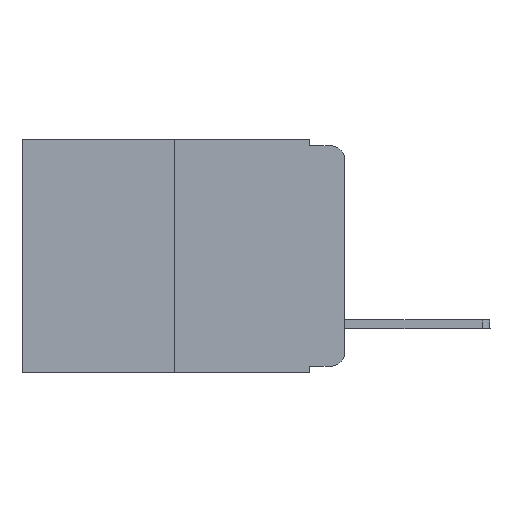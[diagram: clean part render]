
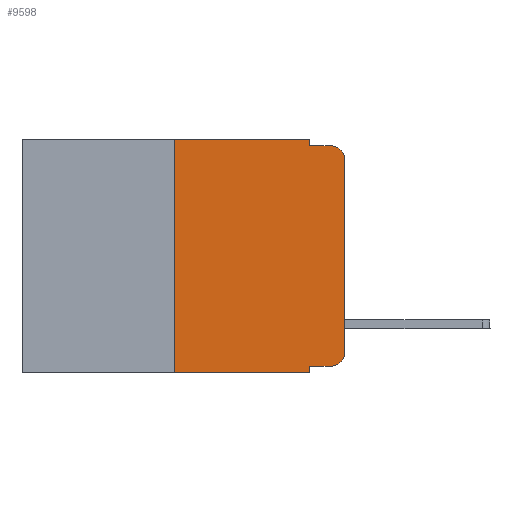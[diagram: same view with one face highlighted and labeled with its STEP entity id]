
A CAD part, left-side view. The second image highlights one B-rep face of the part: STEP entity #9598.
In plain terms, the highlighted planar face has unit normal (-1, 0, 0).
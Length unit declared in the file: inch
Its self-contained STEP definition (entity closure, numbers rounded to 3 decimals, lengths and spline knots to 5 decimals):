
#320 = CARTESIAN_POINT ( 'NONE',  ( 0., 0.02, -0.333 ) ) ;
#509 = ORIENTED_EDGE ( 'NONE', *, *, #8006, .T. ) ;
#600 = DIRECTION ( 'NONE',  ( 0., -1., 0. ) ) ;
#733 = DIRECTION ( 'NONE',  ( 0., 0., 1. ) ) ;
#1272 = AXIS2_PLACEMENT_3D ( 'NONE', #6115, #7047, #1819 ) ;
#1307 = CARTESIAN_POINT ( 'NONE',  ( 0., 0.051, 0. ) ) ;
#1331 = EDGE_CURVE ( 'NONE', #5371, #3654, #4336, .T. ) ;
#1522 = DIRECTION ( 'NONE',  ( 0., -1., 0. ) ) ;
#1611 = EDGE_CURVE ( 'NONE', #2599, #4344, #7031, .T. ) ;
#1660 = CARTESIAN_POINT ( 'NONE',  ( 0., 0.051, -0.01 ) ) ;
#1819 = DIRECTION ( 'NONE',  ( 0., 0., -1. ) ) ;
#1866 = LINE ( 'NONE', #10562, #9379 ) ;
#2234 = DIRECTION ( 'NONE',  ( 1., 0., 0. ) ) ;
#2406 = DIRECTION ( 'NONE',  ( 0., 0., -1. ) ) ;
#2551 = CARTESIAN_POINT ( 'NONE',  ( 0., 0., 0. ) ) ;
#2599 = VERTEX_POINT ( 'NONE', #320 ) ;
#3126 = CARTESIAN_POINT ( 'NONE',  ( 0., 0.473, 0. ) ) ;
#3312 = VECTOR ( 'NONE', #733, 39.37008 ) ;
#3349 = AXIS2_PLACEMENT_3D ( 'NONE', #8077, #9720, #3787 ) ;
#3357 = DIRECTION ( 'NONE',  ( 0., 0., 1. ) ) ;
#3554 = LINE ( 'NONE', #3730, #6795 ) ;
#3560 = EDGE_CURVE ( 'NONE', #9716, #3654, #1866, .T. ) ;
#3654 = VERTEX_POINT ( 'NONE', #4282 ) ;
#3685 = ORIENTED_EDGE ( 'NONE', *, *, #5083, .F. ) ;
#3730 = CARTESIAN_POINT ( 'NONE',  ( 0., 0.051, 0. ) ) ;
#3787 = DIRECTION ( 'NONE',  ( 0., 0., -1. ) ) ;
#3791 = LINE ( 'NONE', #6676, #6636 ) ;
#3878 = FACE_OUTER_BOUND ( 'NONE', #8320, .T. ) ;
#4020 = VECTOR ( 'NONE', #3357, 39.37008 ) ;
#4061 = VERTEX_POINT ( 'NONE', #4195 ) ;
#4195 = CARTESIAN_POINT ( 'NONE',  ( 0., 0.051, -0.333 ) ) ;
#4274 = VERTEX_POINT ( 'NONE', #7795 ) ;
#4282 = CARTESIAN_POINT ( 'NONE',  ( 0., 0.02, -0.01 ) ) ;
#4336 = CIRCLE ( 'NONE', #1272, 0.02 ) ;
#4344 = VERTEX_POINT ( 'NONE', #4670 ) ;
#4571 = CARTESIAN_POINT ( 'NONE',  ( 0., 0.25, -0.343 ) ) ;
#4670 = CARTESIAN_POINT ( 'NONE',  ( 0., 0., -0.313 ) ) ;
#4980 = AXIS2_PLACEMENT_3D ( 'NONE', #3126, #2234, #8237 ) ;
#5061 = EDGE_CURVE ( 'NONE', #5521, #4274, #9986, .T. ) ;
#5083 = EDGE_CURVE ( 'NONE', #4061, #6143, #7874, .T. ) ;
#5113 = VECTOR ( 'NONE', #7084, 39.37008 ) ;
#5371 = VERTEX_POINT ( 'NONE', #5692 ) ;
#5455 = ORIENTED_EDGE ( 'NONE', *, *, #9641, .T. ) ;
#5495 = EDGE_CURVE ( 'NONE', #8202, #9716, #3554, .T. ) ;
#5521 = VERTEX_POINT ( 'NONE', #4571 ) ;
#5579 = VECTOR ( 'NONE', #600, 39.37008 ) ;
#5635 = LINE ( 'NONE', #2551, #4020 ) ;
#5692 = CARTESIAN_POINT ( 'NONE',  ( 0., 0., -0.03 ) ) ;
#6052 = EDGE_CURVE ( 'NONE', #4274, #8202, #8121, .T. ) ;
#6115 = CARTESIAN_POINT ( 'NONE',  ( 0., 0.02, -0.03 ) ) ;
#6143 = VERTEX_POINT ( 'NONE', #6522 ) ;
#6444 = EDGE_CURVE ( 'NONE', #5521, #6143, #3791, .T. ) ;
#6522 = CARTESIAN_POINT ( 'NONE',  ( 0., 0.051, -0.343 ) ) ;
#6524 = CARTESIAN_POINT ( 'NONE',  ( 0., 0.25, 0. ) ) ;
#6636 = VECTOR ( 'NONE', #1522, 39.37008 ) ;
#6676 = CARTESIAN_POINT ( 'NONE',  ( 0., 0.473, -0.343 ) ) ;
#6795 = VECTOR ( 'NONE', #9735, 39.37008 ) ;
#7031 = CIRCLE ( 'NONE', #3349, 0.02 ) ;
#7047 = DIRECTION ( 'NONE',  ( -1., 0., 0. ) ) ;
#7084 = DIRECTION ( 'NONE',  ( 0., -1., 0. ) ) ;
#7347 = VECTOR ( 'NONE', #2406, 39.37008 ) ;
#7387 = PLANE ( 'NONE',  #4980 ) ;
#7670 = ORIENTED_EDGE ( 'NONE', *, *, #5495, .F. ) ;
#7795 = CARTESIAN_POINT ( 'NONE',  ( 0., 0.25, 0. ) ) ;
#7874 = LINE ( 'NONE', #10951, #7347 ) ;
#7905 = CARTESIAN_POINT ( 'NONE',  ( 0., 0.051, -0.333 ) ) ;
#8006 = EDGE_CURVE ( 'NONE', #4061, #2599, #8462, .T. ) ;
#8077 = CARTESIAN_POINT ( 'NONE',  ( 0., 0.02, -0.313 ) ) ;
#8111 = ORIENTED_EDGE ( 'NONE', *, *, #5061, .F. ) ;
#8121 = LINE ( 'NONE', #10791, #5579 ) ;
#8202 = VERTEX_POINT ( 'NONE', #1307 ) ;
#8237 = DIRECTION ( 'NONE',  ( 0., 0., -1. ) ) ;
#8320 = EDGE_LOOP ( 'NONE', ( #5455, #9955, #8497, #7670, #9460, #8111, #9897, #3685, #509, #8425 ) ) ;
#8425 = ORIENTED_EDGE ( 'NONE', *, *, #1611, .T. ) ;
#8462 = LINE ( 'NONE', #7905, #5113 ) ;
#8497 = ORIENTED_EDGE ( 'NONE', *, *, #3560, .F. ) ;
#8925 = DIRECTION ( 'NONE',  ( 0., -1., 0. ) ) ;
#9379 = VECTOR ( 'NONE', #8925, 39.37008 ) ;
#9460 = ORIENTED_EDGE ( 'NONE', *, *, #6052, .F. ) ;
#9598 = ADVANCED_FACE ( 'NONE', ( #3878 ), #7387, .F. ) ;
#9641 = EDGE_CURVE ( 'NONE', #4344, #5371, #5635, .T. ) ;
#9716 = VERTEX_POINT ( 'NONE', #1660 ) ;
#9720 = DIRECTION ( 'NONE',  ( -1., 0., 0. ) ) ;
#9735 = DIRECTION ( 'NONE',  ( 0., 0., -1. ) ) ;
#9897 = ORIENTED_EDGE ( 'NONE', *, *, #6444, .T. ) ;
#9955 = ORIENTED_EDGE ( 'NONE', *, *, #1331, .T. ) ;
#9986 = LINE ( 'NONE', #6524, #3312 ) ;
#10562 = CARTESIAN_POINT ( 'NONE',  ( 0., 0.051, -0.01 ) ) ;
#10791 = CARTESIAN_POINT ( 'NONE',  ( 0., 0.473, 0. ) ) ;
#10951 = CARTESIAN_POINT ( 'NONE',  ( 0., 0.051, 0. ) ) ;
